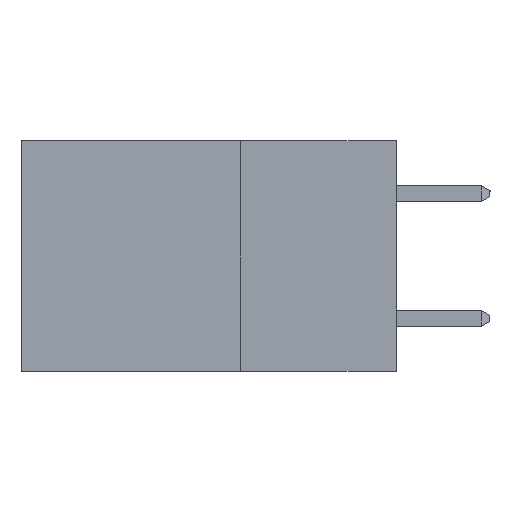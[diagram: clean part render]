
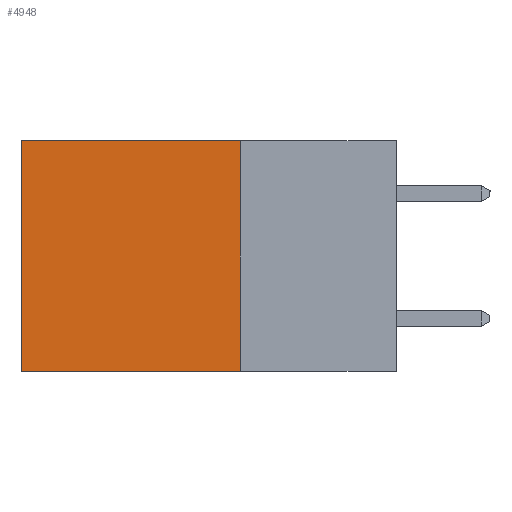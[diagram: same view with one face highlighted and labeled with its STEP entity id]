
A CAD part, left-side view. The second image highlights one B-rep face of the part: STEP entity #4948.
In plain terms, the highlighted planar face has unit normal (-1, 0, 0).
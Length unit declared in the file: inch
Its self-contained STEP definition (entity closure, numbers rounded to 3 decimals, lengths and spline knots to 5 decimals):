
#157 = VECTOR ( 'NONE', #627, 39.37008 ) ;
#563 = DIRECTION ( 'NONE',  ( 1., 0., 0. ) ) ;
#627 = DIRECTION ( 'NONE',  ( 0., 1., 0. ) ) ;
#778 = DIRECTION ( 'NONE',  ( 0., 1., 0. ) ) ;
#865 = CARTESIAN_POINT ( 'NONE',  ( 0.2615, 0.25, 0. ) ) ;
#1366 = VERTEX_POINT ( 'NONE', #3595 ) ;
#1425 = LINE ( 'NONE', #1510, #6006 ) ;
#1444 = LINE ( 'NONE', #4927, #157 ) ;
#1510 = CARTESIAN_POINT ( 'NONE',  ( 0.2615, 0.6, -0.37 ) ) ;
#1515 = EDGE_CURVE ( 'NONE', #6356, #8814, #7092, .T. ) ;
#1648 = VECTOR ( 'NONE', #7420, 39.37008 ) ;
#1949 = VERTEX_POINT ( 'NONE', #5081 ) ;
#2207 = DIRECTION ( 'NONE',  ( 0., 0., -1. ) ) ;
#2286 = EDGE_CURVE ( 'NONE', #6356, #1366, #3788, .T. ) ;
#2521 = EDGE_LOOP ( 'NONE', ( #5502, #5271, #5616, #5177 ) ) ;
#2944 = CARTESIAN_POINT ( 'NONE',  ( 0.2615, 0.25, -0.37 ) ) ;
#2984 = EDGE_CURVE ( 'NONE', #8814, #1949, #1444, .T. ) ;
#3346 = DIRECTION ( 'NONE',  ( 0., 0., -1. ) ) ;
#3518 = CARTESIAN_POINT ( 'NONE',  ( 0.2615, 0.25, -0.37 ) ) ;
#3595 = CARTESIAN_POINT ( 'NONE',  ( 0.2615, 0.6, 0. ) ) ;
#3788 = LINE ( 'NONE', #865, #7725 ) ;
#3927 = EDGE_CURVE ( 'NONE', #1366, #1949, #1425, .T. ) ;
#4243 = CARTESIAN_POINT ( 'NONE',  ( 0.2615, 0.25, 0. ) ) ;
#4927 = CARTESIAN_POINT ( 'NONE',  ( 0.2615, 0.25, -0.37 ) ) ;
#4948 = ADVANCED_FACE ( 'NONE', ( #5464 ), #8384, .F. ) ;
#5081 = CARTESIAN_POINT ( 'NONE',  ( 0.2615, 0.6, -0.37 ) ) ;
#5177 = ORIENTED_EDGE ( 'NONE', *, *, #2286, .T. ) ;
#5271 = ORIENTED_EDGE ( 'NONE', *, *, #2984, .F. ) ;
#5464 = FACE_OUTER_BOUND ( 'NONE', #2521, .T. ) ;
#5502 = ORIENTED_EDGE ( 'NONE', *, *, #3927, .T. ) ;
#5616 = ORIENTED_EDGE ( 'NONE', *, *, #1515, .F. ) ;
#6006 = VECTOR ( 'NONE', #2207, 39.37008 ) ;
#6158 = AXIS2_PLACEMENT_3D ( 'NONE', #3518, #563, #3346 ) ;
#6356 = VERTEX_POINT ( 'NONE', #4243 ) ;
#7092 = LINE ( 'NONE', #2944, #1648 ) ;
#7420 = DIRECTION ( 'NONE',  ( 0., 0., -1. ) ) ;
#7725 = VECTOR ( 'NONE', #778, 39.37008 ) ;
#7794 = CARTESIAN_POINT ( 'NONE',  ( 0.2615, 0.25, -0.37 ) ) ;
#8384 = PLANE ( 'NONE',  #6158 ) ;
#8814 = VERTEX_POINT ( 'NONE', #7794 ) ;
